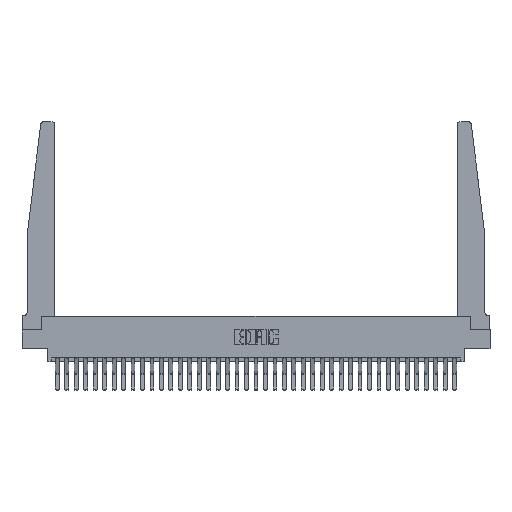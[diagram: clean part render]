
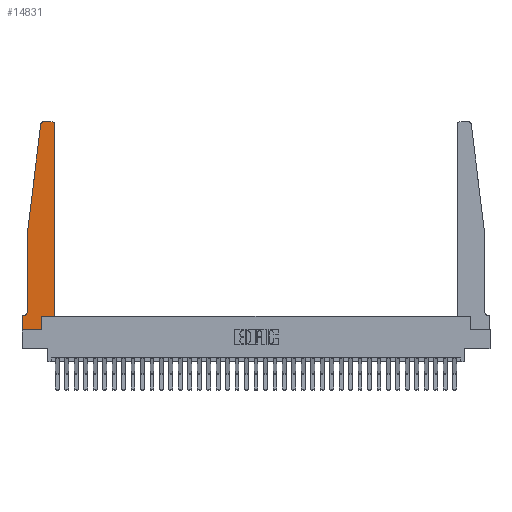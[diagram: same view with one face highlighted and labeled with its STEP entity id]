
A CAD part, top view. The second image highlights one B-rep face of the part: STEP entity #14831.
In plain terms, the highlighted planar face has unit normal (0, 0, 1).
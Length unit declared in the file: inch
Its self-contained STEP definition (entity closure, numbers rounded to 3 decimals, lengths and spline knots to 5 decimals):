
#24 = VERTEX_POINT ( 'NONE', #30130 ) ;
#921 = PLANE ( 'NONE',  #6096 ) ;
#1203 = ORIENTED_EDGE ( 'NONE', *, *, #29847, .T. ) ;
#1700 = CARTESIAN_POINT ( 'NONE',  ( 0.27653, 2.75, 0.37 ) ) ;
#1784 = EDGE_CURVE ( 'NONE', #30452, #18201, #24044, .T. ) ;
#2215 = EDGE_CURVE ( 'NONE', #14980, #15384, #6798, .T. ) ;
#2522 = VERTEX_POINT ( 'NONE', #2682 ) ;
#2682 = CARTESIAN_POINT ( 'NONE',  ( 0.395, 2.75, 0.37 ) ) ;
#2760 = LINE ( 'NONE', #6011, #17171 ) ;
#3639 = CARTESIAN_POINT ( 'NONE',  ( 0.425, 0.18, 0.37 ) ) ;
#3984 = VERTEX_POINT ( 'NONE', #13174 ) ;
#6011 = CARTESIAN_POINT ( 'NONE',  ( 0., 0., 0.37 ) ) ;
#6096 = AXIS2_PLACEMENT_3D ( 'NONE', #21297, #23986, #8659 ) ;
#6097 = VECTOR ( 'NONE', #29604, 39.37008 ) ;
#6172 = CARTESIAN_POINT ( 'NONE',  ( 0.065, 0.2375, 0.37 ) ) ;
#6798 = CIRCLE ( 'NONE', #28762, 0.03 ) ;
#7255 = DIRECTION ( 'NONE',  ( 0., 1., 0. ) ) ;
#7694 = LINE ( 'NONE', #11821, #6097 ) ;
#8280 = CARTESIAN_POINT ( 'NONE',  ( 0.015, 0.2375, 0.37 ) ) ;
#8331 = DIRECTION ( 'NONE',  ( 0., 0., 1. ) ) ;
#8498 = CARTESIAN_POINT ( 'NONE',  ( 0.24675, 2.72367, 0.37 ) ) ;
#8659 = DIRECTION ( 'NONE',  ( 1., 0., 0. ) ) ;
#8732 = CARTESIAN_POINT ( 'NONE',  ( 0.27653, 2.72, 0.37 ) ) ;
#9581 = VERTEX_POINT ( 'NONE', #15694 ) ;
#9648 = ORIENTED_EDGE ( 'NONE', *, *, #14324, .T. ) ;
#9851 = CARTESIAN_POINT ( 'NONE',  ( 0.2605, 0.18, 0.37 ) ) ;
#9871 = LINE ( 'NONE', #9851, #15857 ) ;
#10135 = EDGE_LOOP ( 'NONE', ( #10817, #19221, #20034, #1203, #21625, #15628, #29138, #9648, #17239, #30717, #18848, #26381 ) ) ;
#10817 = ORIENTED_EDGE ( 'NONE', *, *, #11199, .T. ) ;
#10855 = DIRECTION ( 'NONE',  ( -1., 0., 0. ) ) ;
#11199 = EDGE_CURVE ( 'NONE', #2522, #14980, #27047, .T. ) ;
#11276 = VERTEX_POINT ( 'NONE', #20632 ) ;
#11302 = DIRECTION ( 'NONE',  ( 1., 0., 0. ) ) ;
#11413 = VECTOR ( 'NONE', #19069, 39.37008 ) ;
#11821 = CARTESIAN_POINT ( 'NONE',  ( 0., 0., 0.37 ) ) ;
#13174 = CARTESIAN_POINT ( 'NONE',  ( 0.425, 2.72, 0.37 ) ) ;
#13726 = CARTESIAN_POINT ( 'NONE',  ( 0.065, 1.25, 0.37 ) ) ;
#14324 = EDGE_CURVE ( 'NONE', #20005, #11276, #7694, .T. ) ;
#14565 = CARTESIAN_POINT ( 'NONE',  ( 0.065, 1.25, 0.37 ) ) ;
#14831 = ADVANCED_FACE ( 'NONE', ( #26408 ), #921, .T. ) ;
#14980 = VERTEX_POINT ( 'NONE', #1700 ) ;
#15289 = EDGE_CURVE ( 'NONE', #24245, #9581, #20447, .T. ) ;
#15384 = VERTEX_POINT ( 'NONE', #8498 ) ;
#15490 = VECTOR ( 'NONE', #28963, 39.37008 ) ;
#15628 = ORIENTED_EDGE ( 'NONE', *, *, #32813, .T. ) ;
#15694 = CARTESIAN_POINT ( 'NONE',  ( 0.015, 0.1875, 0.37 ) ) ;
#15857 = VECTOR ( 'NONE', #7255, 39.37008 ) ;
#15877 = VECTOR ( 'NONE', #19717, 39.37008 ) ;
#16603 = CARTESIAN_POINT ( 'NONE',  ( 0.425, 0.18, 0.37 ) ) ;
#17171 = VECTOR ( 'NONE', #23930, 39.37008 ) ;
#17232 = VECTOR ( 'NONE', #26817, 39.37008 ) ;
#17239 = ORIENTED_EDGE ( 'NONE', *, *, #26988, .T. ) ;
#17840 = DIRECTION ( 'NONE',  ( -1., 0., 0. ) ) ;
#18201 = VERTEX_POINT ( 'NONE', #18811 ) ;
#18811 = CARTESIAN_POINT ( 'NONE',  ( 0.425, 0.18, 0.37 ) ) ;
#18848 = ORIENTED_EDGE ( 'NONE', *, *, #28647, .T. ) ;
#19069 = DIRECTION ( 'NONE',  ( 0., 1., 0. ) ) ;
#19178 = AXIS2_PLACEMENT_3D ( 'NONE', #8280, #26125, #10855 ) ;
#19221 = ORIENTED_EDGE ( 'NONE', *, *, #2215, .T. ) ;
#19717 = DIRECTION ( 'NONE',  ( -0.122, -0.992, 0. ) ) ;
#20005 = VERTEX_POINT ( 'NONE', #27966 ) ;
#20034 = ORIENTED_EDGE ( 'NONE', *, *, #21234, .T. ) ;
#20447 = CIRCLE ( 'NONE', #19178, 0.05 ) ;
#20632 = CARTESIAN_POINT ( 'NONE',  ( 0.2605, 0., 0.37 ) ) ;
#21234 = EDGE_CURVE ( 'NONE', #15384, #22024, #24293, .T. ) ;
#21297 = CARTESIAN_POINT ( 'NONE',  ( 0., 0.1875, 0.37 ) ) ;
#21413 = CARTESIAN_POINT ( 'NONE',  ( 0.2605, 0.18, 0.37 ) ) ;
#21625 = ORIENTED_EDGE ( 'NONE', *, *, #15289, .T. ) ;
#22024 = VERTEX_POINT ( 'NONE', #22622 ) ;
#22622 = CARTESIAN_POINT ( 'NONE',  ( 0.065, 1.25, 0.37 ) ) ;
#22861 = CARTESIAN_POINT ( 'NONE',  ( 0.25, 2.75, 0.37 ) ) ;
#23679 = CARTESIAN_POINT ( 'NONE',  ( 0.395, 2.72, 0.37 ) ) ;
#23930 = DIRECTION ( 'NONE',  ( 0., -1., 0. ) ) ;
#23986 = DIRECTION ( 'NONE',  ( 0., 0., 1. ) ) ;
#24044 = LINE ( 'NONE', #16603, #17232 ) ;
#24245 = VERTEX_POINT ( 'NONE', #6172 ) ;
#24293 = LINE ( 'NONE', #14565, #15877 ) ;
#25340 = EDGE_CURVE ( 'NONE', #24, #20005, #2760, .T. ) ;
#25784 = LINE ( 'NONE', #3639, #11413 ) ;
#26125 = DIRECTION ( 'NONE',  ( 0., 0., -1. ) ) ;
#26185 = DIRECTION ( 'NONE',  ( 1., 0., 0. ) ) ;
#26381 = ORIENTED_EDGE ( 'NONE', *, *, #31244, .T. ) ;
#26408 = FACE_OUTER_BOUND ( 'NONE', #10135, .T. ) ;
#26438 = LINE ( 'NONE', #27298, #30777 ) ;
#26562 = DIRECTION ( 'NONE',  ( 0., 0., 1. ) ) ;
#26817 = DIRECTION ( 'NONE',  ( 1., 0., 0. ) ) ;
#26988 = EDGE_CURVE ( 'NONE', #11276, #30452, #9871, .T. ) ;
#27047 = LINE ( 'NONE', #22861, #32929 ) ;
#27298 = CARTESIAN_POINT ( 'NONE',  ( 0.065, 0.1875, 0.37 ) ) ;
#27966 = CARTESIAN_POINT ( 'NONE',  ( 0., 0., 0.37 ) ) ;
#28647 = EDGE_CURVE ( 'NONE', #18201, #3984, #25784, .T. ) ;
#28762 = AXIS2_PLACEMENT_3D ( 'NONE', #8732, #26562, #11302 ) ;
#28963 = DIRECTION ( 'NONE',  ( 0., -1., 0. ) ) ;
#29004 = LINE ( 'NONE', #13726, #15490 ) ;
#29138 = ORIENTED_EDGE ( 'NONE', *, *, #25340, .T. ) ;
#29215 = AXIS2_PLACEMENT_3D ( 'NONE', #23679, #8331, #26185 ) ;
#29604 = DIRECTION ( 'NONE',  ( 1., 0., 0. ) ) ;
#29706 = CIRCLE ( 'NONE', #29215, 0.03 ) ;
#29834 = DIRECTION ( 'NONE',  ( -1., 0., 0. ) ) ;
#29847 = EDGE_CURVE ( 'NONE', #22024, #24245, #29004, .T. ) ;
#30130 = CARTESIAN_POINT ( 'NONE',  ( 0., 0.1875, 0.37 ) ) ;
#30452 = VERTEX_POINT ( 'NONE', #21413 ) ;
#30717 = ORIENTED_EDGE ( 'NONE', *, *, #1784, .T. ) ;
#30777 = VECTOR ( 'NONE', #29834, 39.37008 ) ;
#31244 = EDGE_CURVE ( 'NONE', #3984, #2522, #29706, .T. ) ;
#32813 = EDGE_CURVE ( 'NONE', #9581, #24, #26438, .T. ) ;
#32929 = VECTOR ( 'NONE', #17840, 39.37008 ) ;
